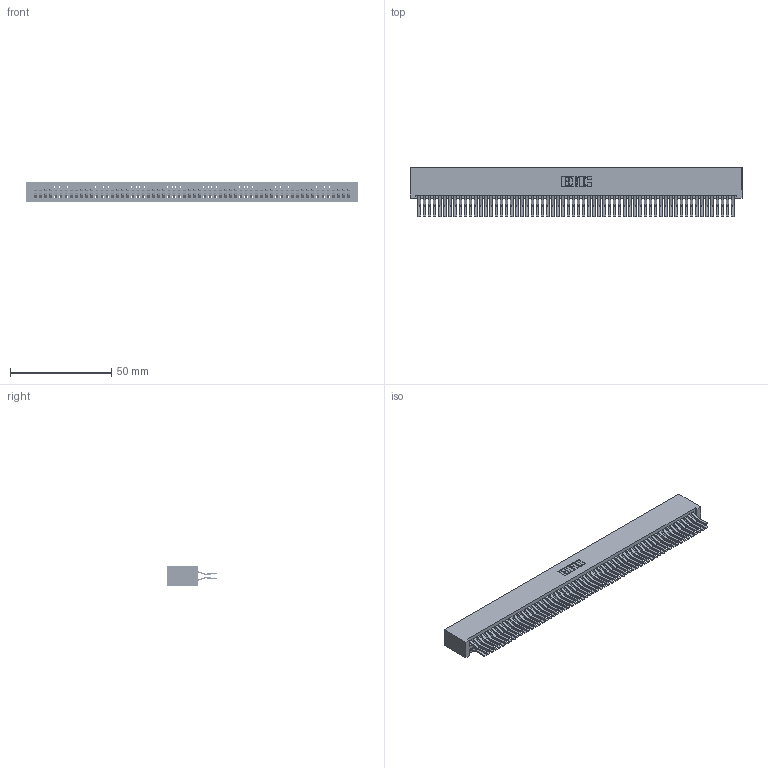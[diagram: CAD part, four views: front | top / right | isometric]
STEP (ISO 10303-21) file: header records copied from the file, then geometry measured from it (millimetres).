
FILE_DESCRIPTION (( 'STEP AP203' ), '1' );
FILE_NAME ('345-124-560-201.STEP', '2018-10-19T11:50:24', ( '' ), ( '' ), 'SwSTEP 2.0', 'SolidWorks 2016', '' );
FILE_SCHEMA (( 'CONFIG_CONTROL_DESIGN' ));
Length unit declared in the file: inch
Products named in the file (3): 345-124-560-201; 345-292-001_560 Tail; 345 Part_No Mounting Lugs
Assembly tree (125 placements, depth 2):
  345-124-560-201
    345 Part_No Mounting Lugs
    345-292-001_560 Tail  x124
Bounding box: 164.08 x 24.45 x 9.4 mm (x, y, z)
Volume: 17553.6 mm3; surface area: 28728.2 mm2
Topology: 125 solids, 125 shells, 6566 faces, 19537 edges, 12858 vertices
Faces by surface type: plane 4168, cylinder 2398
Entity records: 45765 total; most frequent: CARTESIAN_POINT 7652, ORIENTED_EDGE 7586, DIRECTION 6721, EDGE_CURVE 3793, VECTOR 3417, LINE 3417, VERTEX_POINT 2526, AXIS2_PLACEMENT_3D 1652
